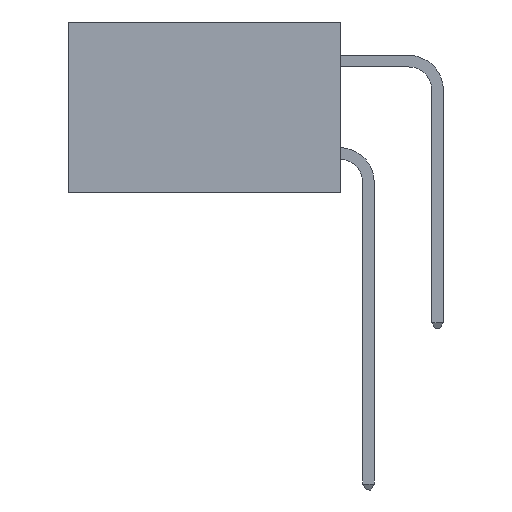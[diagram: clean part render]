
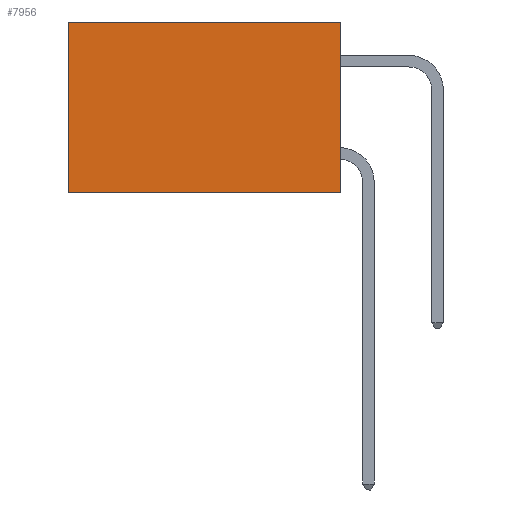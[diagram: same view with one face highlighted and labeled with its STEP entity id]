
A CAD part, left-side view. The second image highlights one B-rep face of the part: STEP entity #7956.
In plain terms, the highlighted planar face has unit normal (-1, 0, 0).
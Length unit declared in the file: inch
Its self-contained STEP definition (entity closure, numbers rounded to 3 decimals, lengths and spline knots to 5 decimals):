
#256 = EDGE_LOOP ( 'NONE', ( #8474, #2646, #7762, #8939 ) ) ;
#422 = CARTESIAN_POINT ( 'NONE',  ( 0.277, 0.59, -0.37 ) ) ;
#997 = VECTOR ( 'NONE', #2828, 39.37008 ) ;
#1205 = VERTEX_POINT ( 'NONE', #422 ) ;
#1428 = CARTESIAN_POINT ( 'NONE',  ( 0.277, 0., -0.37 ) ) ;
#1457 = VECTOR ( 'NONE', #6871, 39.37008 ) ;
#1585 = DIRECTION ( 'NONE',  ( 0., 0., -1. ) ) ;
#1700 = LINE ( 'NONE', #5350, #1457 ) ;
#2152 = CARTESIAN_POINT ( 'NONE',  ( 0.277, 0., 0. ) ) ;
#2405 = CARTESIAN_POINT ( 'NONE',  ( 0.277, 0., -0.37 ) ) ;
#2646 = ORIENTED_EDGE ( 'NONE', *, *, #7212, .F. ) ;
#2828 = DIRECTION ( 'NONE',  ( 0., 1., 0. ) ) ;
#3056 = CARTESIAN_POINT ( 'NONE',  ( 0.277, 0.59, 0. ) ) ;
#3087 = VECTOR ( 'NONE', #7004, 39.37008 ) ;
#3446 = VERTEX_POINT ( 'NONE', #3056 ) ;
#4061 = DIRECTION ( 'NONE',  ( 1., 0., 0. ) ) ;
#4135 = CARTESIAN_POINT ( 'NONE',  ( 0.277, 0., -0.37 ) ) ;
#4198 = LINE ( 'NONE', #7399, #997 ) ;
#4287 = FACE_OUTER_BOUND ( 'NONE', #256, .T. ) ;
#4872 = EDGE_CURVE ( 'NONE', #5102, #7357, #8433, .T. ) ;
#5102 = VERTEX_POINT ( 'NONE', #2152 ) ;
#5206 = EDGE_CURVE ( 'NONE', #3446, #1205, #1700, .T. ) ;
#5320 = AXIS2_PLACEMENT_3D ( 'NONE', #6344, #4061, #9322 ) ;
#5350 = CARTESIAN_POINT ( 'NONE',  ( 0.277, 0.59, -0.37 ) ) ;
#6344 = CARTESIAN_POINT ( 'NONE',  ( 0.277, 0., -0.37 ) ) ;
#6409 = EDGE_CURVE ( 'NONE', #5102, #3446, #4198, .T. ) ;
#6441 = VECTOR ( 'NONE', #1585, 39.37008 ) ;
#6871 = DIRECTION ( 'NONE',  ( 0., 0., -1. ) ) ;
#7004 = DIRECTION ( 'NONE',  ( 0., 1., 0. ) ) ;
#7212 = EDGE_CURVE ( 'NONE', #7357, #1205, #8658, .T. ) ;
#7357 = VERTEX_POINT ( 'NONE', #4135 ) ;
#7399 = CARTESIAN_POINT ( 'NONE',  ( 0.277, 0., 0. ) ) ;
#7762 = ORIENTED_EDGE ( 'NONE', *, *, #4872, .F. ) ;
#7956 = ADVANCED_FACE ( 'NONE', ( #4287 ), #8579, .F. ) ;
#8433 = LINE ( 'NONE', #1428, #6441 ) ;
#8474 = ORIENTED_EDGE ( 'NONE', *, *, #5206, .T. ) ;
#8579 = PLANE ( 'NONE',  #5320 ) ;
#8658 = LINE ( 'NONE', #2405, #3087 ) ;
#8939 = ORIENTED_EDGE ( 'NONE', *, *, #6409, .T. ) ;
#9322 = DIRECTION ( 'NONE',  ( 0., 0., -1. ) ) ;
